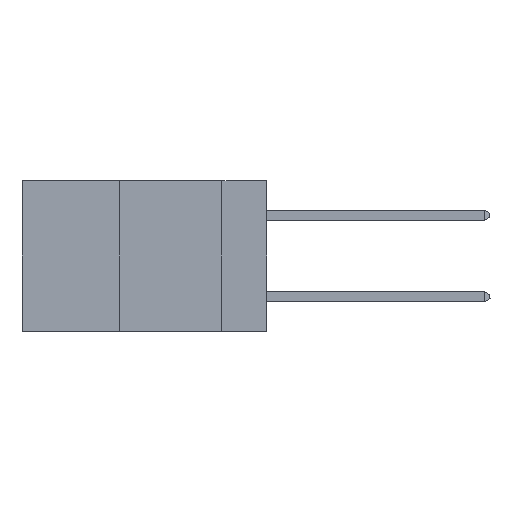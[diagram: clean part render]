
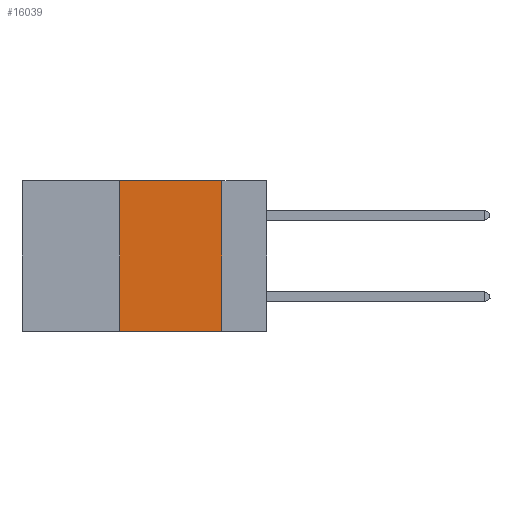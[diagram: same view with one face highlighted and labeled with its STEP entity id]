
A CAD part, left-side view. The second image highlights one B-rep face of the part: STEP entity #16039.
In plain terms, the highlighted planar face has unit normal (-1, 0, 0).
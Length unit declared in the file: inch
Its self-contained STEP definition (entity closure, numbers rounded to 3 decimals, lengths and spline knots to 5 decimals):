
#35 = DIRECTION ( 'NONE',  ( 0., -1., 0. ) ) ;
#288 = DIRECTION ( 'NONE',  ( 0., 0., -1. ) ) ;
#582 = CARTESIAN_POINT ( 'NONE',  ( 0., 0.11, 0. ) ) ;
#612 = CARTESIAN_POINT ( 'NONE',  ( 0., 0.36, 0. ) ) ;
#644 = VERTEX_POINT ( 'NONE', #3591 ) ;
#1258 = CARTESIAN_POINT ( 'NONE',  ( 0., 0.6, 0. ) ) ;
#1403 = DIRECTION ( 'NONE',  ( 1., 0., 0. ) ) ;
#1518 = ORIENTED_EDGE ( 'NONE', *, *, #16740, .F. ) ;
#1870 = ORIENTED_EDGE ( 'NONE', *, *, #13608, .F. ) ;
#3591 = CARTESIAN_POINT ( 'NONE',  ( 0., 0.36, -0.37 ) ) ;
#4506 = AXIS2_PLACEMENT_3D ( 'NONE', #12280, #1403, #288 ) ;
#4787 = EDGE_CURVE ( 'NONE', #644, #9540, #5225, .T. ) ;
#5008 = ORIENTED_EDGE ( 'NONE', *, *, #5198, .F. ) ;
#5198 = EDGE_CURVE ( 'NONE', #10523, #9540, #8558, .T. ) ;
#5225 = LINE ( 'NONE', #16024, #15528 ) ;
#5925 = DIRECTION ( 'NONE',  ( 0., 0., 1. ) ) ;
#6665 = LINE ( 'NONE', #612, #13383 ) ;
#6721 = EDGE_LOOP ( 'NONE', ( #5008, #1518, #1870, #9344 ) ) ;
#8558 = LINE ( 'NONE', #582, #10251 ) ;
#8840 = CARTESIAN_POINT ( 'NONE',  ( 0., 0.36, 0. ) ) ;
#9344 = ORIENTED_EDGE ( 'NONE', *, *, #4787, .T. ) ;
#9540 = VERTEX_POINT ( 'NONE', #13711 ) ;
#10251 = VECTOR ( 'NONE', #15395, 39.37008 ) ;
#10523 = VERTEX_POINT ( 'NONE', #13432 ) ;
#11120 = LINE ( 'NONE', #1258, #13596 ) ;
#12280 = CARTESIAN_POINT ( 'NONE',  ( 0., 0.6, 0. ) ) ;
#12346 = PLANE ( 'NONE',  #4506 ) ;
#13383 = VECTOR ( 'NONE', #5925, 39.37008 ) ;
#13432 = CARTESIAN_POINT ( 'NONE',  ( 0., 0.11, 0. ) ) ;
#13438 = DIRECTION ( 'NONE',  ( 0., -1., 0. ) ) ;
#13572 = VERTEX_POINT ( 'NONE', #8840 ) ;
#13596 = VECTOR ( 'NONE', #35, 39.37008 ) ;
#13608 = EDGE_CURVE ( 'NONE', #644, #13572, #6665, .T. ) ;
#13711 = CARTESIAN_POINT ( 'NONE',  ( 0., 0.11, -0.37 ) ) ;
#14494 = FACE_OUTER_BOUND ( 'NONE', #6721, .T. ) ;
#15395 = DIRECTION ( 'NONE',  ( 0., 0., -1. ) ) ;
#15528 = VECTOR ( 'NONE', #13438, 39.37008 ) ;
#16024 = CARTESIAN_POINT ( 'NONE',  ( 0., 0.6, -0.37 ) ) ;
#16039 = ADVANCED_FACE ( 'NONE', ( #14494 ), #12346, .F. ) ;
#16740 = EDGE_CURVE ( 'NONE', #13572, #10523, #11120, .T. ) ;
